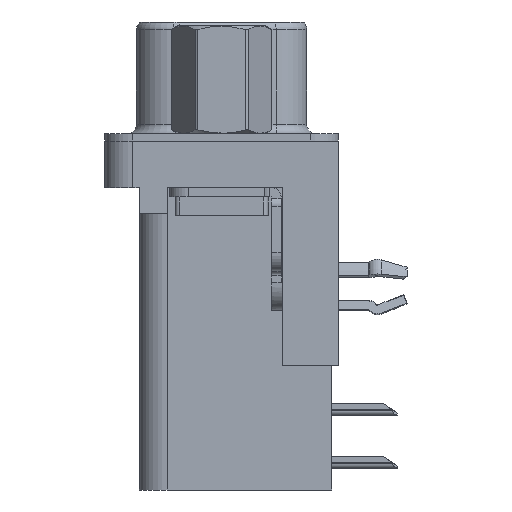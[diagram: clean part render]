
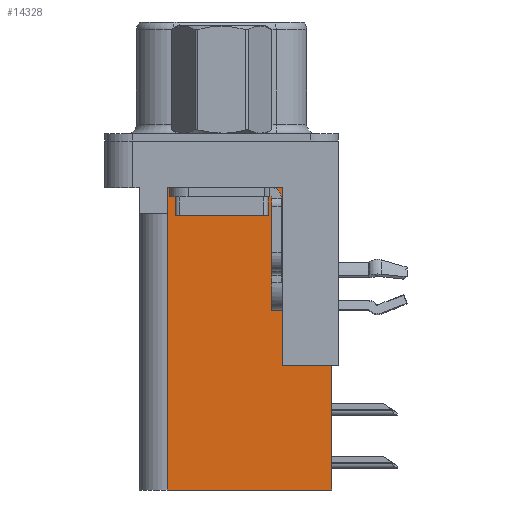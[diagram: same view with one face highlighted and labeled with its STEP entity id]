
A CAD part, left-side view. The second image highlights one B-rep face of the part: STEP entity #14328.
In plain terms, the highlighted planar face has unit normal (-1, 0, 0).
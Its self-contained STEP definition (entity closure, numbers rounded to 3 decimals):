
#211 = EDGE_LOOP ( 'NONE', ( #17871, #19140, #1518, #5987, #28161, #21632, #23708, #9178 ) ) ;
#1320 = VERTEX_POINT ( 'NONE', #20983 ) ;
#1336 = CARTESIAN_POINT ( 'NONE',  ( 3.79, -5.925, -18.76 ) ) ;
#1518 = ORIENTED_EDGE ( 'NONE', *, *, #10399, .T. ) ;
#1855 = DIRECTION ( 'NONE',  ( 0., 1., 0. ) ) ;
#2922 = CARTESIAN_POINT ( 'NONE',  ( 3.79, 2.925, -18.76 ) ) ;
#3325 = CARTESIAN_POINT ( 'NONE',  ( 3.79, -5.925, -2. ) ) ;
#3409 = VECTOR ( 'NONE', #26401, 1000. ) ;
#3827 = LINE ( 'NONE', #2922, #3409 ) ;
#4132 = EDGE_CURVE ( 'NONE', #1320, #13198, #3827, .T. ) ;
#5717 = EDGE_CURVE ( 'NONE', #11506, #25451, #24595, .T. ) ;
#5788 = VECTOR ( 'NONE', #22515, 1000. ) ;
#5821 = LINE ( 'NONE', #32549, #5788 ) ;
#5987 = ORIENTED_EDGE ( 'NONE', *, *, #4132, .F. ) ;
#6873 = VERTEX_POINT ( 'NONE', #7155 ) ;
#7155 = CARTESIAN_POINT ( 'NONE',  ( 3.79, -3.295, -12.05 ) ) ;
#7850 = DIRECTION ( 'NONE',  ( 0., 0., 1. ) ) ;
#8158 = CARTESIAN_POINT ( 'NONE',  ( 3.79, 2.925, -3.9 ) ) ;
#8224 = EDGE_CURVE ( 'NONE', #25451, #8261, #5821, .T. ) ;
#8261 = VERTEX_POINT ( 'NONE', #32646 ) ;
#8714 = DIRECTION ( 'NONE',  ( 0., 1., 0. ) ) ;
#9178 = ORIENTED_EDGE ( 'NONE', *, *, #31691, .T. ) ;
#10007 = LINE ( 'NONE', #30425, #10071 ) ;
#10071 = VECTOR ( 'NONE', #32845, 1000. ) ;
#10399 = EDGE_CURVE ( 'NONE', #8261, #13198, #13879, .T. ) ;
#11506 = VERTEX_POINT ( 'NONE', #16225 ) ;
#12017 = AXIS2_PLACEMENT_3D ( 'NONE', #31774, #24280, #8714 ) ;
#12022 = DIRECTION ( 'NONE',  ( 0., 1., 0. ) ) ;
#13198 = VERTEX_POINT ( 'NONE', #8158 ) ;
#13640 = VECTOR ( 'NONE', #31289, 1000. ) ;
#13879 = LINE ( 'NONE', #15838, #13640 ) ;
#14032 = VERTEX_POINT ( 'NONE', #1336 ) ;
#14328 = ADVANCED_FACE ( 'NONE', ( #30157 ), #21592, .F. ) ;
#15838 = CARTESIAN_POINT ( 'NONE',  ( 3.79, 0., -3.9 ) ) ;
#16113 = CARTESIAN_POINT ( 'NONE',  ( 3.79, 2.895, -2.5 ) ) ;
#16225 = CARTESIAN_POINT ( 'NONE',  ( 3.79, -3.295, -2.5 ) ) ;
#16289 = DIRECTION ( 'NONE',  ( 0., 0., -1. ) ) ;
#17553 = CARTESIAN_POINT ( 'NONE',  ( 3.79, -3.295, -2.5 ) ) ;
#17871 = ORIENTED_EDGE ( 'NONE', *, *, #5717, .T. ) ;
#19140 = ORIENTED_EDGE ( 'NONE', *, *, #8224, .T. ) ;
#20588 = VECTOR ( 'NONE', #16289, 1000. ) ;
#20713 = LINE ( 'NONE', #3325, #20588 ) ;
#20983 = CARTESIAN_POINT ( 'NONE',  ( 3.79, 2.925, -18.76 ) ) ;
#21335 = VECTOR ( 'NONE', #12022, 1000. ) ;
#21592 = PLANE ( 'NONE',  #12017 ) ;
#21632 = ORIENTED_EDGE ( 'NONE', *, *, #26454, .F. ) ;
#22515 = DIRECTION ( 'NONE',  ( 0., 0., -1. ) ) ;
#22543 = EDGE_CURVE ( 'NONE', #14032, #1320, #23359, .T. ) ;
#23359 = LINE ( 'NONE', #30074, #21335 ) ;
#23420 = CARTESIAN_POINT ( 'NONE',  ( 3.79, -3.295, -18.76 ) ) ;
#23708 = ORIENTED_EDGE ( 'NONE', *, *, #29352, .T. ) ;
#24280 = DIRECTION ( 'NONE',  ( 1., 0., 0. ) ) ;
#24577 = CARTESIAN_POINT ( 'NONE',  ( 3.79, -5.925, -12.05 ) ) ;
#24595 = LINE ( 'NONE', #17553, #24956 ) ;
#24956 = VECTOR ( 'NONE', #1855, 1000. ) ;
#25451 = VERTEX_POINT ( 'NONE', #16113 ) ;
#26401 = DIRECTION ( 'NONE',  ( 0., 0., 1. ) ) ;
#26454 = EDGE_CURVE ( 'NONE', #27166, #14032, #20713, .T. ) ;
#27166 = VERTEX_POINT ( 'NONE', #24577 ) ;
#28161 = ORIENTED_EDGE ( 'NONE', *, *, #22543, .F. ) ;
#29352 = EDGE_CURVE ( 'NONE', #27166, #6873, #10007, .T. ) ;
#30074 = CARTESIAN_POINT ( 'NONE',  ( 3.79, -3.295, -18.76 ) ) ;
#30157 = FACE_OUTER_BOUND ( 'NONE', #211, .T. ) ;
#30425 = CARTESIAN_POINT ( 'NONE',  ( 3.79, -6.295, -12.05 ) ) ;
#30612 = VECTOR ( 'NONE', #7850, 1000. ) ;
#30914 = LINE ( 'NONE', #23420, #30612 ) ;
#31289 = DIRECTION ( 'NONE',  ( 0., 1., 0. ) ) ;
#31691 = EDGE_CURVE ( 'NONE', #6873, #11506, #30914, .T. ) ;
#31774 = CARTESIAN_POINT ( 'NONE',  ( 3.79, -3.295, -18.76 ) ) ;
#32549 = CARTESIAN_POINT ( 'NONE',  ( 3.79, 2.895, -3.9 ) ) ;
#32646 = CARTESIAN_POINT ( 'NONE',  ( 3.79, 2.895, -3.9 ) ) ;
#32845 = DIRECTION ( 'NONE',  ( 0., 1., 0. ) ) ;
